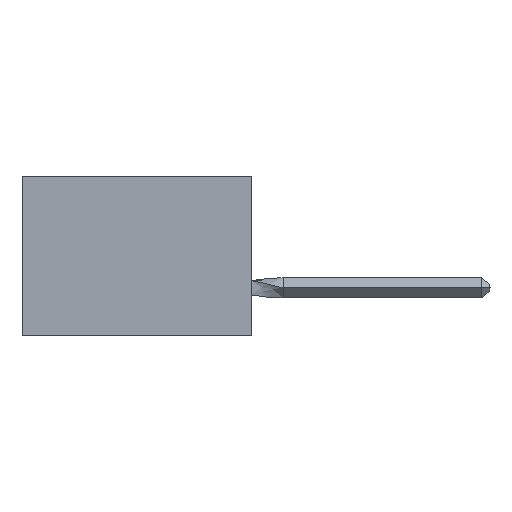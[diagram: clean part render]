
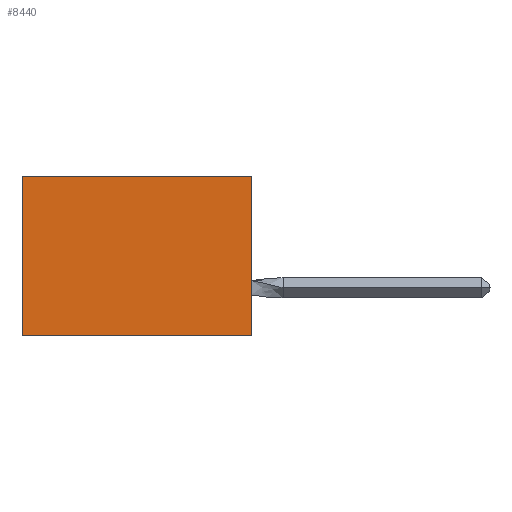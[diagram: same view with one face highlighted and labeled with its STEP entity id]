
A CAD part, left-side view. The second image highlights one B-rep face of the part: STEP entity #8440.
In plain terms, the highlighted planar face has unit normal (-1, 0, 0).
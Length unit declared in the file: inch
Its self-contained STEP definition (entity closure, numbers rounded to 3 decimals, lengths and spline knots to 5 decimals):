
#300 = EDGE_CURVE ( 'NONE', #8329, #18362, #15006, .T. ) ;
#873 = FACE_OUTER_BOUND ( 'NONE', #5982, .T. ) ;
#897 = CARTESIAN_POINT ( 'NONE',  ( 0.305, 0., 0. ) ) ;
#1271 = DIRECTION ( 'NONE',  ( 0., 1., 0. ) ) ;
#1507 = CARTESIAN_POINT ( 'NONE',  ( 0.305, 0., -0.5 ) ) ;
#1587 = LINE ( 'NONE', #2961, #12479 ) ;
#1661 = LINE ( 'NONE', #17904, #4116 ) ;
#1686 = CARTESIAN_POINT ( 'NONE',  ( 0.305, 0.72, 0. ) ) ;
#1816 = ORIENTED_EDGE ( 'NONE', *, *, #300, .F. ) ;
#2646 = CARTESIAN_POINT ( 'NONE',  ( 0.305, 0., -0.5 ) ) ;
#2961 = CARTESIAN_POINT ( 'NONE',  ( 0.305, 0.72, -0.5 ) ) ;
#3541 = ORIENTED_EDGE ( 'NONE', *, *, #7326, .T. ) ;
#4116 = VECTOR ( 'NONE', #16589, 39.37008 ) ;
#4336 = DIRECTION ( 'NONE',  ( 0., 0., -1. ) ) ;
#5790 = PLANE ( 'NONE',  #15032 ) ;
#5910 = DIRECTION ( 'NONE',  ( 0., 0., -1. ) ) ;
#5982 = EDGE_LOOP ( 'NONE', ( #16628, #1816, #8016, #3541 ) ) ;
#7311 = EDGE_CURVE ( 'NONE', #9807, #8329, #1661, .T. ) ;
#7326 = EDGE_CURVE ( 'NONE', #9807, #11076, #16340, .T. ) ;
#7692 = VECTOR ( 'NONE', #7971, 39.37008 ) ;
#7971 = DIRECTION ( 'NONE',  ( 0., 1., 0. ) ) ;
#8016 = ORIENTED_EDGE ( 'NONE', *, *, #7311, .F. ) ;
#8329 = VERTEX_POINT ( 'NONE', #2646 ) ;
#8440 = ADVANCED_FACE ( 'NONE', ( #873 ), #5790, .F. ) ;
#9807 = VERTEX_POINT ( 'NONE', #897 ) ;
#9816 = CARTESIAN_POINT ( 'NONE',  ( 0.305, 0., -0.5 ) ) ;
#11076 = VERTEX_POINT ( 'NONE', #1686 ) ;
#12479 = VECTOR ( 'NONE', #5910, 39.37008 ) ;
#13885 = CARTESIAN_POINT ( 'NONE',  ( 0.305, 0.72, -0.5 ) ) ;
#15006 = LINE ( 'NONE', #9816, #15911 ) ;
#15032 = AXIS2_PLACEMENT_3D ( 'NONE', #1507, #15694, #4336 ) ;
#15694 = DIRECTION ( 'NONE',  ( 1., 0., 0. ) ) ;
#15911 = VECTOR ( 'NONE', #1271, 39.37008 ) ;
#16340 = LINE ( 'NONE', #16400, #7692 ) ;
#16400 = CARTESIAN_POINT ( 'NONE',  ( 0.305, 0., 0. ) ) ;
#16589 = DIRECTION ( 'NONE',  ( 0., 0., -1. ) ) ;
#16628 = ORIENTED_EDGE ( 'NONE', *, *, #16767, .T. ) ;
#16767 = EDGE_CURVE ( 'NONE', #11076, #18362, #1587, .T. ) ;
#17904 = CARTESIAN_POINT ( 'NONE',  ( 0.305, 0., -0.5 ) ) ;
#18362 = VERTEX_POINT ( 'NONE', #13885 ) ;
